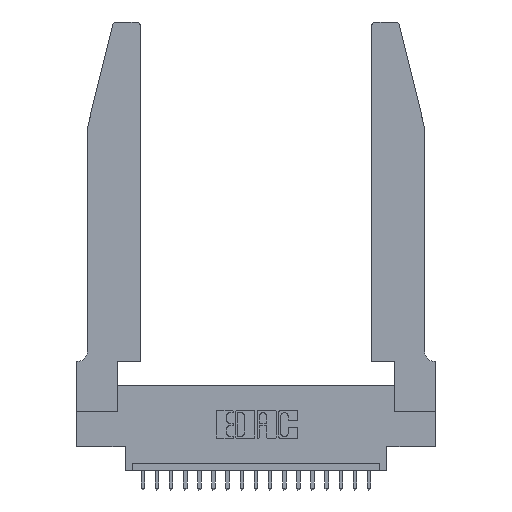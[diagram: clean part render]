
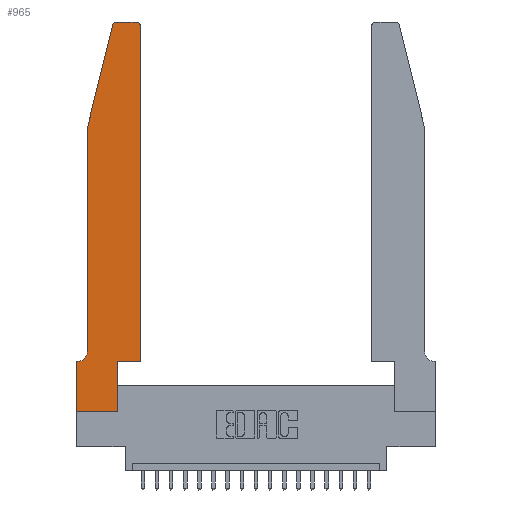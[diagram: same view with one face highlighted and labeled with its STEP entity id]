
A CAD part, top view. The second image highlights one B-rep face of the part: STEP entity #965.
In plain terms, the highlighted planar face has unit normal (0, 0, 1).
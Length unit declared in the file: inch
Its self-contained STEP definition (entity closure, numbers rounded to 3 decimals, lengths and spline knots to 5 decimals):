
#150 = ORIENTED_EDGE ( 'NONE', *, *, #2800, .T. ) ;
#177 = ORIENTED_EDGE ( 'NONE', *, *, #8576, .T. ) ;
#363 = CIRCLE ( 'NONE', #20369, 0.03 ) ;
#450 = CARTESIAN_POINT ( 'NONE',  ( 0.25487, 2.72718, 0.37 ) ) ;
#482 = CARTESIAN_POINT ( 'NONE',  ( 0.0755, 0.35, 0.37 ) ) ;
#644 = CARTESIAN_POINT ( 'NONE',  ( 0.0055, 0.42, 0.37 ) ) ;
#856 = ORIENTED_EDGE ( 'NONE', *, *, #16525, .T. ) ;
#965 = ADVANCED_FACE ( 'NONE', ( #19795 ), #985, .T. ) ;
#985 = PLANE ( 'NONE',  #8828 ) ;
#1085 = ORIENTED_EDGE ( 'NONE', *, *, #2210, .T. ) ;
#1404 = LINE ( 'NONE', #9218, #7505 ) ;
#1781 = ORIENTED_EDGE ( 'NONE', *, *, #9822, .T. ) ;
#1792 = DIRECTION ( 'NONE',  ( 0., 0., 1. ) ) ;
#1793 = ORIENTED_EDGE ( 'NONE', *, *, #5617, .T. ) ;
#1870 = DIRECTION ( 'NONE',  ( 0., -1., 0. ) ) ;
#2087 = LINE ( 'NONE', #482, #6924 ) ;
#2210 = EDGE_CURVE ( 'NONE', #6469, #8389, #19223, .T. ) ;
#2800 = EDGE_CURVE ( 'NONE', #4022, #17274, #363, .T. ) ;
#3385 = EDGE_CURVE ( 'NONE', #17274, #8726, #3681, .T. ) ;
#3681 = LINE ( 'NONE', #5770, #6479 ) ;
#3694 = EDGE_CURVE ( 'NONE', #18838, #18120, #20465, .T. ) ;
#4022 = VERTEX_POINT ( 'NONE', #15741 ) ;
#4376 = ORIENTED_EDGE ( 'NONE', *, *, #7586, .T. ) ;
#4460 = CARTESIAN_POINT ( 'NONE',  ( 0.2865, 0.35, 0.37 ) ) ;
#4846 = EDGE_CURVE ( 'NONE', #18593, #7361, #8842, .T. ) ;
#5516 = AXIS2_PLACEMENT_3D ( 'NONE', #644, #20415, #10457 ) ;
#5617 = EDGE_CURVE ( 'NONE', #8389, #11898, #1404, .T. ) ;
#5699 = VECTOR ( 'NONE', #7020, 39.37008 ) ;
#5770 = CARTESIAN_POINT ( 'NONE',  ( 0.2605, 2.75, 0.37 ) ) ;
#6120 = EDGE_CURVE ( 'NONE', #18120, #4022, #8273, .T. ) ;
#6469 = VERTEX_POINT ( 'NONE', #15980 ) ;
#6479 = VECTOR ( 'NONE', #17174, 39.37008 ) ;
#6632 = CARTESIAN_POINT ( 'NONE',  ( 0.0755, 2., 0.37 ) ) ;
#6910 = CARTESIAN_POINT ( 'NONE',  ( 0.4505, 0.35, 0.37 ) ) ;
#6924 = VECTOR ( 'NONE', #18427, 39.37008 ) ;
#7020 = DIRECTION ( 'NONE',  ( 0., 1., 0. ) ) ;
#7043 = CARTESIAN_POINT ( 'NONE',  ( 0.4505, 0.35, 0.37 ) ) ;
#7327 = CARTESIAN_POINT ( 'NONE',  ( 0.0755, 0.42, 0.37 ) ) ;
#7361 = VERTEX_POINT ( 'NONE', #9057 ) ;
#7505 = VECTOR ( 'NONE', #11057, 39.37008 ) ;
#7586 = EDGE_CURVE ( 'NONE', #7361, #6469, #2087, .T. ) ;
#7891 = ORIENTED_EDGE ( 'NONE', *, *, #4846, .T. ) ;
#8138 = CIRCLE ( 'NONE', #12143, 0.03 ) ;
#8266 = VECTOR ( 'NONE', #12114, 39.37008 ) ;
#8273 = LINE ( 'NONE', #15157, #5699 ) ;
#8389 = VERTEX_POINT ( 'NONE', #9763 ) ;
#8576 = EDGE_CURVE ( 'NONE', #11898, #18838, #11725, .T. ) ;
#8726 = VERTEX_POINT ( 'NONE', #14635 ) ;
#8792 = VECTOR ( 'NONE', #14224, 39.37008 ) ;
#8818 = CARTESIAN_POINT ( 'NONE',  ( 0., 0.35, 0.37 ) ) ;
#8828 = AXIS2_PLACEMENT_3D ( 'NONE', #8818, #9098, #8890 ) ;
#8842 = CIRCLE ( 'NONE', #5516, 0.07 ) ;
#8890 = DIRECTION ( 'NONE',  ( 1., 0., 0. ) ) ;
#9057 = CARTESIAN_POINT ( 'NONE',  ( 0.0055, 0.35, 0.37 ) ) ;
#9098 = DIRECTION ( 'NONE',  ( 0., 0., 1. ) ) ;
#9218 = CARTESIAN_POINT ( 'NONE',  ( 0., 0., 0.37 ) ) ;
#9311 = DIRECTION ( 'NONE',  ( 1., 0., 0. ) ) ;
#9763 = CARTESIAN_POINT ( 'NONE',  ( 0., 0., 0.37 ) ) ;
#9822 = EDGE_CURVE ( 'NONE', #8726, #16793, #8138, .T. ) ;
#10457 = DIRECTION ( 'NONE',  ( -1., 0., 0. ) ) ;
#11057 = DIRECTION ( 'NONE',  ( 1., 0., 0. ) ) ;
#11214 = VECTOR ( 'NONE', #13800, 39.37008 ) ;
#11481 = ORIENTED_EDGE ( 'NONE', *, *, #3694, .T. ) ;
#11725 = LINE ( 'NONE', #11886, #11214 ) ;
#11886 = CARTESIAN_POINT ( 'NONE',  ( 0.2865, 0.35, 0.37 ) ) ;
#11898 = VERTEX_POINT ( 'NONE', #17549 ) ;
#12114 = DIRECTION ( 'NONE',  ( -0.239, -0.971, 0. ) ) ;
#12143 = AXIS2_PLACEMENT_3D ( 'NONE', #14313, #1792, #13304 ) ;
#12376 = CARTESIAN_POINT ( 'NONE',  ( 0.4205, 2.72, 0.37 ) ) ;
#12442 = VECTOR ( 'NONE', #13177, 39.37008 ) ;
#12459 = CARTESIAN_POINT ( 'NONE',  ( 0., 0., 0.37 ) ) ;
#12620 = CARTESIAN_POINT ( 'NONE',  ( 0.0755, 2., 0.37 ) ) ;
#12788 = ORIENTED_EDGE ( 'NONE', *, *, #3385, .T. ) ;
#13177 = DIRECTION ( 'NONE',  ( 1., 0., 0. ) ) ;
#13304 = DIRECTION ( 'NONE',  ( 1., 0., 0. ) ) ;
#13755 = ORIENTED_EDGE ( 'NONE', *, *, #19630, .T. ) ;
#13800 = DIRECTION ( 'NONE',  ( 0., 1., 0. ) ) ;
#13824 = EDGE_LOOP ( 'NONE', ( #12788, #1781, #856, #13755, #7891, #4376, #1085, #1793, #177, #11481, #17939, #150 ) ) ;
#14224 = DIRECTION ( 'NONE',  ( 0., -1., 0. ) ) ;
#14313 = CARTESIAN_POINT ( 'NONE',  ( 0.284, 2.72, 0.37 ) ) ;
#14635 = CARTESIAN_POINT ( 'NONE',  ( 0.284, 2.75, 0.37 ) ) ;
#15157 = CARTESIAN_POINT ( 'NONE',  ( 0.4505, 0.35, 0.37 ) ) ;
#15604 = CARTESIAN_POINT ( 'NONE',  ( 0.0755, 2., 0.37 ) ) ;
#15741 = CARTESIAN_POINT ( 'NONE',  ( 0.4505, 2.72, 0.37 ) ) ;
#15980 = CARTESIAN_POINT ( 'NONE',  ( 0., 0.35, 0.37 ) ) ;
#16410 = LINE ( 'NONE', #15604, #8266 ) ;
#16525 = EDGE_CURVE ( 'NONE', #16793, #19480, #16410, .T. ) ;
#16729 = VECTOR ( 'NONE', #1870, 39.37008 ) ;
#16793 = VERTEX_POINT ( 'NONE', #450 ) ;
#17174 = DIRECTION ( 'NONE',  ( -1., 0., 0. ) ) ;
#17274 = VERTEX_POINT ( 'NONE', #19806 ) ;
#17549 = CARTESIAN_POINT ( 'NONE',  ( 0.2865, 0., 0.37 ) ) ;
#17939 = ORIENTED_EDGE ( 'NONE', *, *, #6120, .T. ) ;
#18120 = VERTEX_POINT ( 'NONE', #7043 ) ;
#18427 = DIRECTION ( 'NONE',  ( -1., 0., 0. ) ) ;
#18593 = VERTEX_POINT ( 'NONE', #7327 ) ;
#18838 = VERTEX_POINT ( 'NONE', #4460 ) ;
#19059 = DIRECTION ( 'NONE',  ( 0., 0., 1. ) ) ;
#19223 = LINE ( 'NONE', #12459, #8792 ) ;
#19480 = VERTEX_POINT ( 'NONE', #12620 ) ;
#19630 = EDGE_CURVE ( 'NONE', #19480, #18593, #21043, .T. ) ;
#19795 = FACE_OUTER_BOUND ( 'NONE', #13824, .T. ) ;
#19806 = CARTESIAN_POINT ( 'NONE',  ( 0.4205, 2.75, 0.37 ) ) ;
#20369 = AXIS2_PLACEMENT_3D ( 'NONE', #12376, #19059, #9311 ) ;
#20415 = DIRECTION ( 'NONE',  ( 0., 0., -1. ) ) ;
#20465 = LINE ( 'NONE', #6910, #12442 ) ;
#21043 = LINE ( 'NONE', #6632, #16729 ) ;
